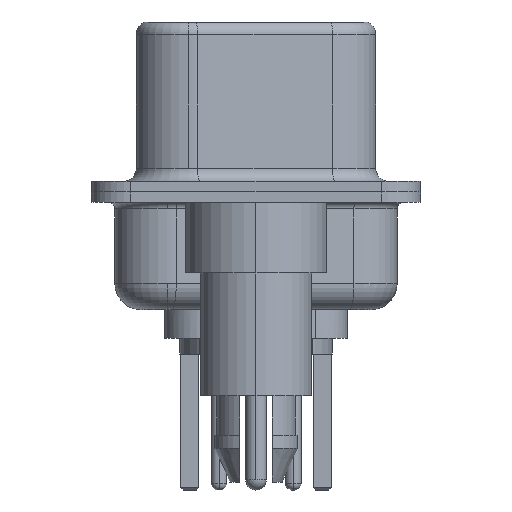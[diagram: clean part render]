
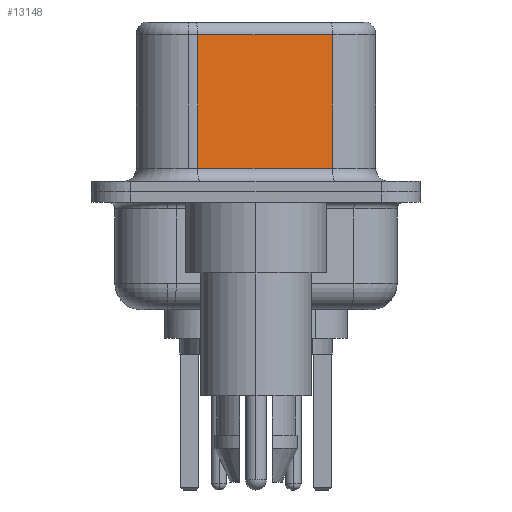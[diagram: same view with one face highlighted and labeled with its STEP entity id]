
A CAD part, left-side view. The second image highlights one B-rep face of the part: STEP entity #13148.
In plain terms, the highlighted planar face has unit normal (-0.985, -0.174, 0).
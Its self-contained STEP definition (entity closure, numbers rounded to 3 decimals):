
#624 = VERTEX_POINT ( 'NONE', #17778 ) ;
#888 = CARTESIAN_POINT ( 'NONE',  ( 4.565, -2.927, 6.52 ) ) ;
#1199 = LINE ( 'NONE', #10472, #13334 ) ;
#1289 = VECTOR ( 'NONE', #2823, 1000. ) ;
#1651 = EDGE_LOOP ( 'NONE', ( #7533, #10829, #6894, #13352 ) ) ;
#2036 = LINE ( 'NONE', #19714, #18498 ) ;
#2823 = DIRECTION ( 'NONE',  ( -0.174, 0.985, 0. ) ) ;
#3689 = VERTEX_POINT ( 'NONE', #10855 ) ;
#3810 = DIRECTION ( 'NONE',  ( 0., 0., -1. ) ) ;
#4007 = DIRECTION ( 'NONE',  ( -0.174, 0.985, 0. ) ) ;
#5213 = CARTESIAN_POINT ( 'NONE',  ( 4.565, -2.927, 0.9 ) ) ;
#5441 = CARTESIAN_POINT ( 'NONE',  ( 4.565, -2.927, 0.9 ) ) ;
#6346 = AXIS2_PLACEMENT_3D ( 'NONE', #888, #13565, #4007 ) ;
#6536 = EDGE_CURVE ( 'NONE', #3689, #11176, #1199, .T. ) ;
#6894 = ORIENTED_EDGE ( 'NONE', *, *, #14066, .T. ) ;
#7533 = ORIENTED_EDGE ( 'NONE', *, *, #6536, .F. ) ;
#7618 = EDGE_CURVE ( 'NONE', #624, #11176, #15025, .T. ) ;
#8257 = EDGE_CURVE ( 'NONE', #3689, #13176, #9676, .T. ) ;
#9235 = CARTESIAN_POINT ( 'NONE',  ( 4.565, -2.927, 6.02 ) ) ;
#9676 = LINE ( 'NONE', #9235, #1289 ) ;
#10334 = DIRECTION ( 'NONE',  ( 0., 0., -1. ) ) ;
#10336 = PLANE ( 'NONE',  #6346 ) ;
#10472 = CARTESIAN_POINT ( 'NONE',  ( 4.565, -2.927, 6.52 ) ) ;
#10801 = VECTOR ( 'NONE', #14953, 1000. ) ;
#10829 = ORIENTED_EDGE ( 'NONE', *, *, #8257, .T. ) ;
#10855 = CARTESIAN_POINT ( 'NONE',  ( 4.565, -2.927, 6.02 ) ) ;
#11176 = VERTEX_POINT ( 'NONE', #5213 ) ;
#12047 = CARTESIAN_POINT ( 'NONE',  ( 3.655, 2.233, 6.02 ) ) ;
#13148 = ADVANCED_FACE ( 'NONE', ( #14034 ), #10336, .F. ) ;
#13176 = VERTEX_POINT ( 'NONE', #12047 ) ;
#13334 = VECTOR ( 'NONE', #10334, 1000. ) ;
#13352 = ORIENTED_EDGE ( 'NONE', *, *, #7618, .T. ) ;
#13565 = DIRECTION ( 'NONE',  ( 0.985, 0.174, 0. ) ) ;
#14034 = FACE_OUTER_BOUND ( 'NONE', #1651, .T. ) ;
#14066 = EDGE_CURVE ( 'NONE', #13176, #624, #2036, .T. ) ;
#14953 = DIRECTION ( 'NONE',  ( 0.174, -0.985, 0. ) ) ;
#15025 = LINE ( 'NONE', #5441, #10801 ) ;
#17778 = CARTESIAN_POINT ( 'NONE',  ( 3.655, 2.233, 0.9 ) ) ;
#18498 = VECTOR ( 'NONE', #3810, 1000. ) ;
#19714 = CARTESIAN_POINT ( 'NONE',  ( 3.655, 2.233, 6.52 ) ) ;
